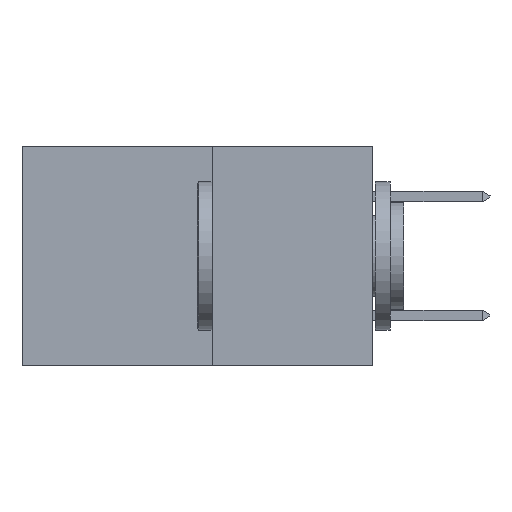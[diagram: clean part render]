
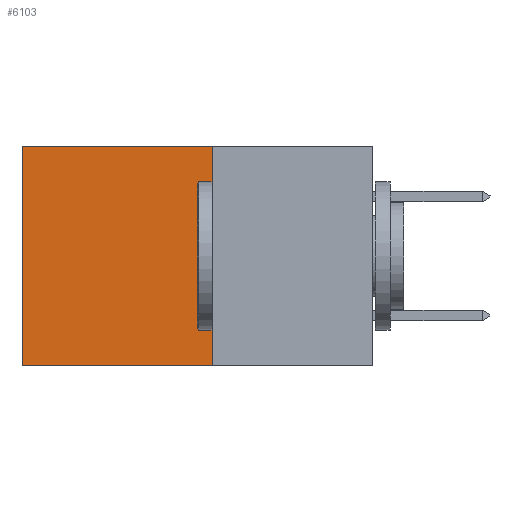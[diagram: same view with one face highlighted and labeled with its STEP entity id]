
A CAD part, left-side view. The second image highlights one B-rep face of the part: STEP entity #6103.
In plain terms, the highlighted planar face has unit normal (-1, 0, 0).
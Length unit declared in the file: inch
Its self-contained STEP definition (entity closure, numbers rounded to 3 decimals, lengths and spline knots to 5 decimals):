
#1200 = CARTESIAN_POINT ( 'NONE',  ( 0.277, 0.59, -0.37 ) ) ;
#1455 = LINE ( 'NONE', #1200, #21728 ) ;
#2350 = LINE ( 'NONE', #21168, #17930 ) ;
#2731 = FACE_OUTER_BOUND ( 'NONE', #24349, .T. ) ;
#2983 = ORIENTED_EDGE ( 'NONE', *, *, #7265, .F. ) ;
#4125 = ORIENTED_EDGE ( 'NONE', *, *, #4658, .F. ) ;
#4347 = DIRECTION ( 'NONE',  ( 0., 0., -1. ) ) ;
#4433 = DIRECTION ( 'NONE',  ( 1., 0., 0. ) ) ;
#4524 = CARTESIAN_POINT ( 'NONE',  ( 0.277, 0.27, -0.37 ) ) ;
#4658 = EDGE_CURVE ( 'NONE', #15835, #6590, #16748, .T. ) ;
#5214 = PLANE ( 'NONE',  #7881 ) ;
#6103 = ADVANCED_FACE ( 'NONE', ( #2731 ), #5214, .F. ) ;
#6590 = VERTEX_POINT ( 'NONE', #22458 ) ;
#7265 = EDGE_CURVE ( 'NONE', #17132, #15835, #2350, .T. ) ;
#7270 = CARTESIAN_POINT ( 'NONE',  ( 0.277, 0.27, 0. ) ) ;
#7881 = AXIS2_PLACEMENT_3D ( 'NONE', #4524, #4433, #4347 ) ;
#10169 = VECTOR ( 'NONE', #10759, 39.37008 ) ;
#10759 = DIRECTION ( 'NONE',  ( 0., 1., 0. ) ) ;
#10838 = CARTESIAN_POINT ( 'NONE',  ( 0.277, 0.59, 0. ) ) ;
#10902 = CARTESIAN_POINT ( 'NONE',  ( 0.277, 0.27, -0.37 ) ) ;
#11162 = CARTESIAN_POINT ( 'NONE',  ( 0.277, 0.27, 0. ) ) ;
#11487 = DIRECTION ( 'NONE',  ( 0., 0., -1. ) ) ;
#13514 = EDGE_CURVE ( 'NONE', #20874, #6590, #1455, .T. ) ;
#15134 = CARTESIAN_POINT ( 'NONE',  ( 0.277, 0.27, -0.37 ) ) ;
#15626 = LINE ( 'NONE', #7270, #20906 ) ;
#15835 = VERTEX_POINT ( 'NONE', #15134 ) ;
#16748 = LINE ( 'NONE', #10902, #10169 ) ;
#17132 = VERTEX_POINT ( 'NONE', #11162 ) ;
#17389 = DIRECTION ( 'NONE',  ( 0., 1., 0. ) ) ;
#17510 = ORIENTED_EDGE ( 'NONE', *, *, #13514, .T. ) ;
#17930 = VECTOR ( 'NONE', #20369, 39.37008 ) ;
#19025 = EDGE_CURVE ( 'NONE', #17132, #20874, #15626, .T. ) ;
#20369 = DIRECTION ( 'NONE',  ( 0., 0., -1. ) ) ;
#20791 = ORIENTED_EDGE ( 'NONE', *, *, #19025, .T. ) ;
#20874 = VERTEX_POINT ( 'NONE', #10838 ) ;
#20906 = VECTOR ( 'NONE', #17389, 39.37008 ) ;
#21168 = CARTESIAN_POINT ( 'NONE',  ( 0.277, 0.27, -0.37 ) ) ;
#21728 = VECTOR ( 'NONE', #11487, 39.37008 ) ;
#22458 = CARTESIAN_POINT ( 'NONE',  ( 0.277, 0.59, -0.37 ) ) ;
#24349 = EDGE_LOOP ( 'NONE', ( #17510, #4125, #2983, #20791 ) ) ;
